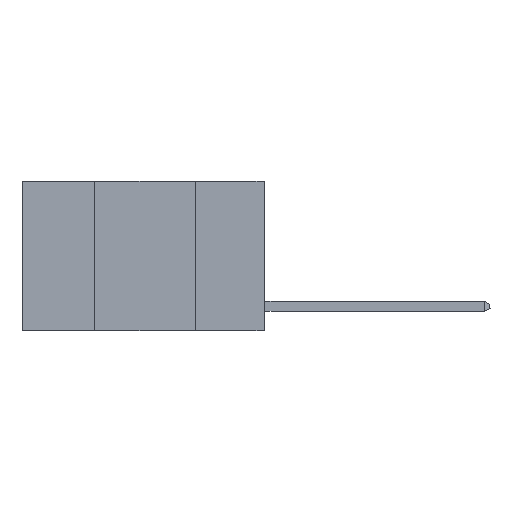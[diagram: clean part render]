
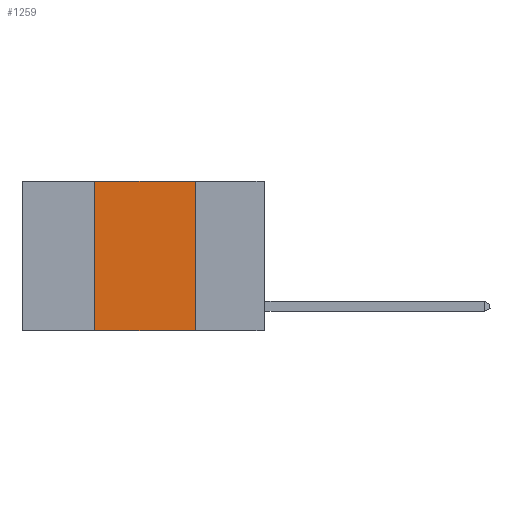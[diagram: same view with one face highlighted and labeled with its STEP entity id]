
A CAD part, left-side view. The second image highlights one B-rep face of the part: STEP entity #1259.
In plain terms, the highlighted planar face has unit normal (-1, 0, 0).
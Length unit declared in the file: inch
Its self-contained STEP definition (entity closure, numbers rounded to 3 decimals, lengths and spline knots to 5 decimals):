
#178 = CARTESIAN_POINT ( 'NONE',  ( 0., 0.6, 0. ) ) ;
#203 = DIRECTION ( 'NONE',  ( 0., -1., 0. ) ) ;
#299 = DIRECTION ( 'NONE',  ( 1., 0., 0. ) ) ;
#325 = CARTESIAN_POINT ( 'NONE',  ( 0., 0.42, -0.37 ) ) ;
#448 = LINE ( 'NONE', #3115, #7704 ) ;
#559 = CARTESIAN_POINT ( 'NONE',  ( 0., 0.17, 0. ) ) ;
#880 = CARTESIAN_POINT ( 'NONE',  ( 0., 0.6, 0. ) ) ;
#1259 = ADVANCED_FACE ( 'NONE', ( #2964 ), #6908, .F. ) ;
#1539 = ORIENTED_EDGE ( 'NONE', *, *, #4779, .F. ) ;
#1565 = VERTEX_POINT ( 'NONE', #325 ) ;
#1696 = CARTESIAN_POINT ( 'NONE',  ( 0., 0.17, -0.37 ) ) ;
#2288 = ORIENTED_EDGE ( 'NONE', *, *, #7655, .F. ) ;
#2471 = VECTOR ( 'NONE', #203, 39.37008 ) ;
#2561 = CARTESIAN_POINT ( 'NONE',  ( 0., 0.17, 0. ) ) ;
#2771 = EDGE_LOOP ( 'NONE', ( #1539, #2288, #5781, #5976 ) ) ;
#2868 = EDGE_CURVE ( 'NONE', #1565, #7541, #3031, .T. ) ;
#2964 = FACE_OUTER_BOUND ( 'NONE', #2771, .T. ) ;
#3031 = LINE ( 'NONE', #3518, #6304 ) ;
#3115 = CARTESIAN_POINT ( 'NONE',  ( 0., 0.42, 0. ) ) ;
#3518 = CARTESIAN_POINT ( 'NONE',  ( 0., 0.6, -0.37 ) ) ;
#3865 = LINE ( 'NONE', #559, #4235 ) ;
#4235 = VECTOR ( 'NONE', #5939, 39.37008 ) ;
#4239 = LINE ( 'NONE', #880, #2471 ) ;
#4264 = CARTESIAN_POINT ( 'NONE',  ( 0., 0.42, 0. ) ) ;
#4779 = EDGE_CURVE ( 'NONE', #5304, #7541, #3865, .T. ) ;
#5179 = AXIS2_PLACEMENT_3D ( 'NONE', #178, #299, #7556 ) ;
#5304 = VERTEX_POINT ( 'NONE', #2561 ) ;
#5542 = DIRECTION ( 'NONE',  ( 0., -1., 0. ) ) ;
#5776 = DIRECTION ( 'NONE',  ( 0., 0., 1. ) ) ;
#5781 = ORIENTED_EDGE ( 'NONE', *, *, #7845, .F. ) ;
#5939 = DIRECTION ( 'NONE',  ( 0., 0., -1. ) ) ;
#5976 = ORIENTED_EDGE ( 'NONE', *, *, #2868, .T. ) ;
#6304 = VECTOR ( 'NONE', #5542, 39.37008 ) ;
#6783 = VERTEX_POINT ( 'NONE', #4264 ) ;
#6908 = PLANE ( 'NONE',  #5179 ) ;
#7541 = VERTEX_POINT ( 'NONE', #1696 ) ;
#7556 = DIRECTION ( 'NONE',  ( 0., 0., -1. ) ) ;
#7655 = EDGE_CURVE ( 'NONE', #6783, #5304, #4239, .T. ) ;
#7704 = VECTOR ( 'NONE', #5776, 39.37008 ) ;
#7845 = EDGE_CURVE ( 'NONE', #1565, #6783, #448, .T. ) ;
